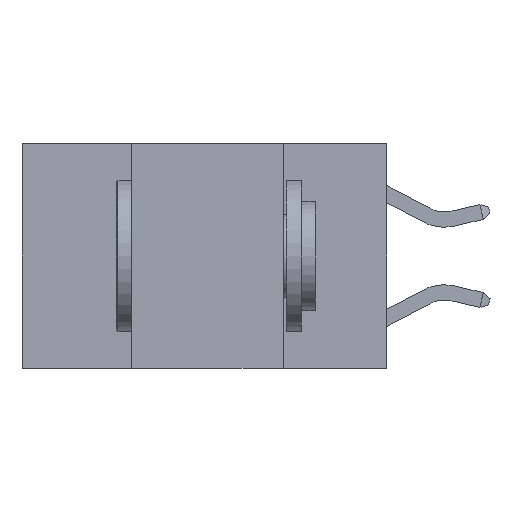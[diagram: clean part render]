
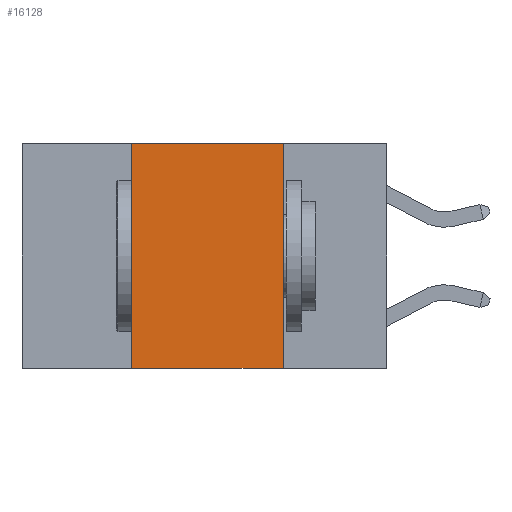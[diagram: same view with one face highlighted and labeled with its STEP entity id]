
A CAD part, left-side view. The second image highlights one B-rep face of the part: STEP entity #16128.
In plain terms, the highlighted planar face has unit normal (-1, 0, 0).
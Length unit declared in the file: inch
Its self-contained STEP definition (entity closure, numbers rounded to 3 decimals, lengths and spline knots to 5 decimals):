
#1794 = LINE ( 'NONE', #7025, #6150 ) ;
#1979 = LINE ( 'NONE', #5170, #6335 ) ;
#4049 = DIRECTION ( 'NONE',  ( 0., -1., 0. ) ) ;
#4183 = VECTOR ( 'NONE', #14115, 39.37008 ) ;
#4216 = ORIENTED_EDGE ( 'NONE', *, *, #4978, .F. ) ;
#4978 = EDGE_CURVE ( 'NONE', #14575, #8691, #1794, .T. ) ;
#5117 = CARTESIAN_POINT ( 'NONE',  ( 0., 0.42, -0.37 ) ) ;
#5170 = CARTESIAN_POINT ( 'NONE',  ( 0., 0.42, 0. ) ) ;
#6150 = VECTOR ( 'NONE', #13781, 39.37008 ) ;
#6335 = VECTOR ( 'NONE', #6918, 39.37008 ) ;
#6506 = EDGE_CURVE ( 'NONE', #21277, #7258, #15592, .T. ) ;
#6918 = DIRECTION ( 'NONE',  ( 0., 0., 1. ) ) ;
#7025 = CARTESIAN_POINT ( 'NONE',  ( 0., 0.6, 0. ) ) ;
#7145 = PLANE ( 'NONE',  #17487 ) ;
#7258 = VERTEX_POINT ( 'NONE', #7445 ) ;
#7445 = CARTESIAN_POINT ( 'NONE',  ( 0., 0.17, -0.37 ) ) ;
#7794 = ORIENTED_EDGE ( 'NONE', *, *, #13974, .F. ) ;
#8691 = VERTEX_POINT ( 'NONE', #18860 ) ;
#8805 = LINE ( 'NONE', #20731, #4183 ) ;
#8825 = DIRECTION ( 'NONE',  ( 1., 0., 0. ) ) ;
#10607 = FACE_OUTER_BOUND ( 'NONE', #17573, .T. ) ;
#13781 = DIRECTION ( 'NONE',  ( 0., -1., 0. ) ) ;
#13837 = ORIENTED_EDGE ( 'NONE', *, *, #22061, .F. ) ;
#13974 = EDGE_CURVE ( 'NONE', #8691, #7258, #8805, .T. ) ;
#14115 = DIRECTION ( 'NONE',  ( 0., 0., -1. ) ) ;
#14575 = VERTEX_POINT ( 'NONE', #21999 ) ;
#15592 = LINE ( 'NONE', #15959, #19994 ) ;
#15959 = CARTESIAN_POINT ( 'NONE',  ( 0., 0.6, -0.37 ) ) ;
#16128 = ADVANCED_FACE ( 'NONE', ( #10607 ), #7145, .F. ) ;
#17487 = AXIS2_PLACEMENT_3D ( 'NONE', #18836, #8825, #20507 ) ;
#17573 = EDGE_LOOP ( 'NONE', ( #7794, #4216, #13837, #18774 ) ) ;
#18774 = ORIENTED_EDGE ( 'NONE', *, *, #6506, .T. ) ;
#18836 = CARTESIAN_POINT ( 'NONE',  ( 0., 0.6, 0. ) ) ;
#18860 = CARTESIAN_POINT ( 'NONE',  ( 0., 0.17, 0. ) ) ;
#19994 = VECTOR ( 'NONE', #4049, 39.37008 ) ;
#20507 = DIRECTION ( 'NONE',  ( 0., 0., -1. ) ) ;
#20731 = CARTESIAN_POINT ( 'NONE',  ( 0., 0.17, 0. ) ) ;
#21277 = VERTEX_POINT ( 'NONE', #5117 ) ;
#21999 = CARTESIAN_POINT ( 'NONE',  ( 0., 0.42, 0. ) ) ;
#22061 = EDGE_CURVE ( 'NONE', #21277, #14575, #1979, .T. ) ;
